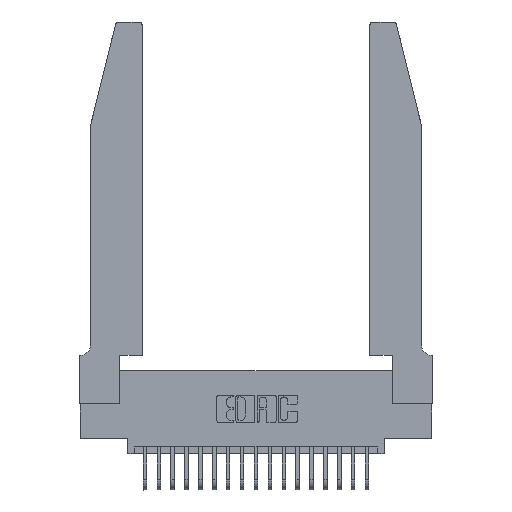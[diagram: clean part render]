
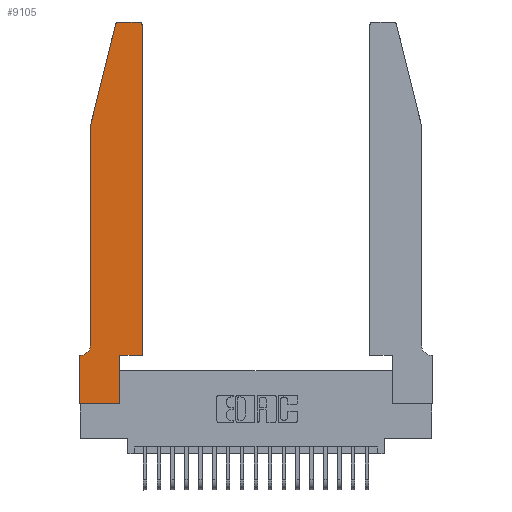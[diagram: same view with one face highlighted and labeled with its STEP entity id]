
A CAD part, top view. The second image highlights one B-rep face of the part: STEP entity #9105.
In plain terms, the highlighted planar face has unit normal (0, 0, 1).
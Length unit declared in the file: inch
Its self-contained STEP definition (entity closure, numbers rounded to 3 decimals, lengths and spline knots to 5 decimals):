
#26 = ORIENTED_EDGE ( 'NONE', *, *, #15120, .T. ) ;
#47 = AXIS2_PLACEMENT_3D ( 'NONE', #8951, #20063, #10545 ) ;
#116 = VECTOR ( 'NONE', #2369, 39.37008 ) ;
#699 = LINE ( 'NONE', #860, #9146 ) ;
#860 = CARTESIAN_POINT ( 'NONE',  ( 0.0755, 0.35, 0.37 ) ) ;
#1823 = VERTEX_POINT ( 'NONE', #11834 ) ;
#1892 = AXIS2_PLACEMENT_3D ( 'NONE', #18964, #9447, #20551 ) ;
#1907 = CARTESIAN_POINT ( 'NONE',  ( 0., 0.35, 0.37 ) ) ;
#2021 = AXIS2_PLACEMENT_3D ( 'NONE', #14533, #4907, #16144 ) ;
#2061 = VERTEX_POINT ( 'NONE', #7553 ) ;
#2161 = ORIENTED_EDGE ( 'NONE', *, *, #14457, .T. ) ;
#2218 = CARTESIAN_POINT ( 'NONE',  ( 0.2865, 0.35, 0.37 ) ) ;
#2369 = DIRECTION ( 'NONE',  ( 1., 0., 0. ) ) ;
#2630 = DIRECTION ( 'NONE',  ( -1., 0., 0. ) ) ;
#2822 = DIRECTION ( 'NONE',  ( -0.239, -0.971, 0. ) ) ;
#2847 = LINE ( 'NONE', #9423, #19039 ) ;
#2962 = EDGE_CURVE ( 'NONE', #19832, #3917, #17979, .T. ) ;
#3502 = ORIENTED_EDGE ( 'NONE', *, *, #14166, .T. ) ;
#3906 = PLANE ( 'NONE',  #19484 ) ;
#3917 = VERTEX_POINT ( 'NONE', #12699 ) ;
#3940 = CIRCLE ( 'NONE', #1892, 0.03 ) ;
#4907 = DIRECTION ( 'NONE',  ( 0., 0., -1. ) ) ;
#4954 = ORIENTED_EDGE ( 'NONE', *, *, #8280, .T. ) ;
#5185 = ORIENTED_EDGE ( 'NONE', *, *, #16738, .T. ) ;
#5829 = CARTESIAN_POINT ( 'NONE',  ( 0.0755, 2., 0.37 ) ) ;
#5925 = VECTOR ( 'NONE', #2822, 39.37008 ) ;
#6522 = ORIENTED_EDGE ( 'NONE', *, *, #12278, .T. ) ;
#7276 = DIRECTION ( 'NONE',  ( 0., 0., 1. ) ) ;
#7528 = VERTEX_POINT ( 'NONE', #1907 ) ;
#7553 = CARTESIAN_POINT ( 'NONE',  ( 0.2865, 0.35, 0.37 ) ) ;
#7591 = LINE ( 'NONE', #20209, #116 ) ;
#7667 = CARTESIAN_POINT ( 'NONE',  ( 0.4505, 0.35, 0.37 ) ) ;
#8043 = LINE ( 'NONE', #7667, #16504 ) ;
#8280 = EDGE_CURVE ( 'NONE', #12371, #11717, #19644, .T. ) ;
#8504 = CIRCLE ( 'NONE', #47, 0.03 ) ;
#8951 = CARTESIAN_POINT ( 'NONE',  ( 0.4205, 2.72, 0.37 ) ) ;
#9105 = ADVANCED_FACE ( 'NONE', ( #17379 ), #3906, .T. ) ;
#9146 = VECTOR ( 'NONE', #2630, 39.37008 ) ;
#9214 = DIRECTION ( 'NONE',  ( -1., 0., 0. ) ) ;
#9221 = ORIENTED_EDGE ( 'NONE', *, *, #15674, .T. ) ;
#9243 = CARTESIAN_POINT ( 'NONE',  ( 0.25487, 2.72718, 0.37 ) ) ;
#9376 = CARTESIAN_POINT ( 'NONE',  ( 0.0755, 0.42, 0.37 ) ) ;
#9423 = CARTESIAN_POINT ( 'NONE',  ( 0., 0., 0.37 ) ) ;
#9426 = CARTESIAN_POINT ( 'NONE',  ( 0.0755, 2., 0.37 ) ) ;
#9447 = DIRECTION ( 'NONE',  ( 0., 0., 1. ) ) ;
#9493 = DIRECTION ( 'NONE',  ( 0., -1., 0. ) ) ;
#10545 = DIRECTION ( 'NONE',  ( 1., 0., 0. ) ) ;
#11045 = ORIENTED_EDGE ( 'NONE', *, *, #19848, .T. ) ;
#11178 = CARTESIAN_POINT ( 'NONE',  ( 0.284, 2.75, 0.37 ) ) ;
#11190 = VERTEX_POINT ( 'NONE', #13192 ) ;
#11402 = EDGE_CURVE ( 'NONE', #16143, #11190, #8504, .T. ) ;
#11528 = DIRECTION ( 'NONE',  ( 1., 0., 0. ) ) ;
#11717 = VERTEX_POINT ( 'NONE', #9376 ) ;
#11792 = VERTEX_POINT ( 'NONE', #11178 ) ;
#11834 = CARTESIAN_POINT ( 'NONE',  ( 0.4505, 0.35, 0.37 ) ) ;
#12079 = DIRECTION ( 'NONE',  ( 0., 1., 0. ) ) ;
#12197 = VECTOR ( 'NONE', #9214, 39.37008 ) ;
#12278 = EDGE_CURVE ( 'NONE', #11190, #11792, #16415, .T. ) ;
#12346 = EDGE_LOOP ( 'NONE', ( #6522, #26, #11045, #4954, #3502, #2161, #9221, #20657, #13696, #20927, #5185, #16232 ) ) ;
#12371 = VERTEX_POINT ( 'NONE', #9426 ) ;
#12629 = CARTESIAN_POINT ( 'NONE',  ( 0., 0., 0.37 ) ) ;
#12699 = CARTESIAN_POINT ( 'NONE',  ( 0.2865, 0., 0.37 ) ) ;
#12739 = VECTOR ( 'NONE', #11528, 39.37008 ) ;
#13192 = CARTESIAN_POINT ( 'NONE',  ( 0.4205, 2.75, 0.37 ) ) ;
#13646 = CARTESIAN_POINT ( 'NONE',  ( 0.0055, 0.35, 0.37 ) ) ;
#13696 = ORIENTED_EDGE ( 'NONE', *, *, #18001, .T. ) ;
#13715 = VECTOR ( 'NONE', #12079, 39.37008 ) ;
#14060 = DIRECTION ( 'NONE',  ( 0., 1., 0. ) ) ;
#14100 = CIRCLE ( 'NONE', #2021, 0.07 ) ;
#14166 = EDGE_CURVE ( 'NONE', #11717, #17993, #14100, .T. ) ;
#14203 = CARTESIAN_POINT ( 'NONE',  ( 0.0755, 2., 0.37 ) ) ;
#14457 = EDGE_CURVE ( 'NONE', #17993, #7528, #699, .T. ) ;
#14533 = CARTESIAN_POINT ( 'NONE',  ( 0.0055, 0.42, 0.37 ) ) ;
#15014 = EDGE_CURVE ( 'NONE', #2061, #1823, #7591, .T. ) ;
#15120 = EDGE_CURVE ( 'NONE', #11792, #16692, #3940, .T. ) ;
#15413 = DIRECTION ( 'NONE',  ( 0., -1., 0. ) ) ;
#15516 = CARTESIAN_POINT ( 'NONE',  ( 0.2605, 2.75, 0.37 ) ) ;
#15674 = EDGE_CURVE ( 'NONE', #7528, #19832, #2847, .T. ) ;
#15904 = VECTOR ( 'NONE', #15413, 39.37008 ) ;
#16143 = VERTEX_POINT ( 'NONE', #20516 ) ;
#16144 = DIRECTION ( 'NONE',  ( -1., 0., 0. ) ) ;
#16232 = ORIENTED_EDGE ( 'NONE', *, *, #11402, .T. ) ;
#16415 = LINE ( 'NONE', #15516, #12197 ) ;
#16504 = VECTOR ( 'NONE', #14060, 39.37008 ) ;
#16692 = VERTEX_POINT ( 'NONE', #9243 ) ;
#16738 = EDGE_CURVE ( 'NONE', #1823, #16143, #8043, .T. ) ;
#16817 = CARTESIAN_POINT ( 'NONE',  ( 0., 0.35, 0.37 ) ) ;
#17379 = FACE_OUTER_BOUND ( 'NONE', #12346, .T. ) ;
#17979 = LINE ( 'NONE', #21023, #12739 ) ;
#17983 = LINE ( 'NONE', #2218, #13715 ) ;
#17993 = VERTEX_POINT ( 'NONE', #13646 ) ;
#18001 = EDGE_CURVE ( 'NONE', #3917, #2061, #17983, .T. ) ;
#18433 = DIRECTION ( 'NONE',  ( 1., 0., 0. ) ) ;
#18685 = LINE ( 'NONE', #14203, #5925 ) ;
#18964 = CARTESIAN_POINT ( 'NONE',  ( 0.284, 2.72, 0.37 ) ) ;
#19039 = VECTOR ( 'NONE', #9493, 39.37008 ) ;
#19484 = AXIS2_PLACEMENT_3D ( 'NONE', #16817, #7276, #18433 ) ;
#19644 = LINE ( 'NONE', #5829, #15904 ) ;
#19832 = VERTEX_POINT ( 'NONE', #12629 ) ;
#19848 = EDGE_CURVE ( 'NONE', #16692, #12371, #18685, .T. ) ;
#20063 = DIRECTION ( 'NONE',  ( 0., 0., 1. ) ) ;
#20209 = CARTESIAN_POINT ( 'NONE',  ( 0.4505, 0.35, 0.37 ) ) ;
#20516 = CARTESIAN_POINT ( 'NONE',  ( 0.4505, 2.72, 0.37 ) ) ;
#20551 = DIRECTION ( 'NONE',  ( 1., 0., 0. ) ) ;
#20657 = ORIENTED_EDGE ( 'NONE', *, *, #2962, .T. ) ;
#20927 = ORIENTED_EDGE ( 'NONE', *, *, #15014, .T. ) ;
#21023 = CARTESIAN_POINT ( 'NONE',  ( 0., 0., 0.37 ) ) ;
